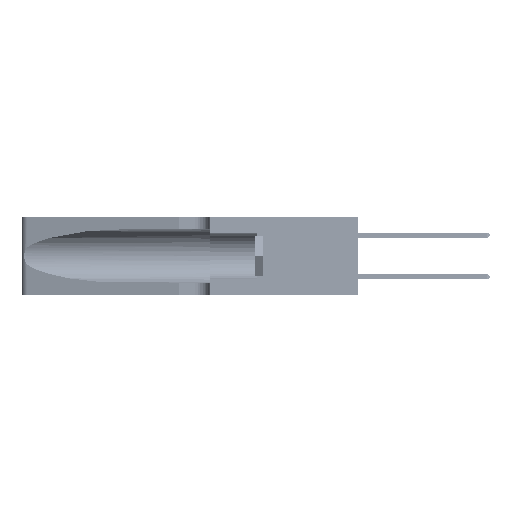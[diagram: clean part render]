
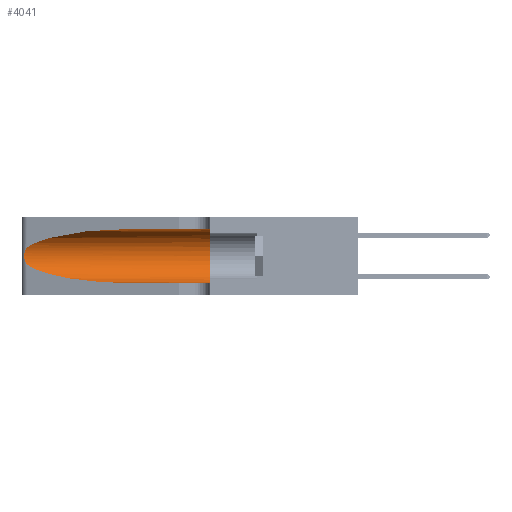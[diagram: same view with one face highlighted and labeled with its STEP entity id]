
A CAD part, left-side view. The second image highlights one B-rep face of the part: STEP entity #4041.
In plain terms, the highlighted cylindrical face has radius 3.308 mm (diameter 6.617 mm), a partial arc.
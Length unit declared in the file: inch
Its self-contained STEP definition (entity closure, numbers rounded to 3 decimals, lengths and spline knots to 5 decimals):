
#20 = DIRECTION ( 'NONE',  ( 0., 0., -1. ) ) ;
#2064 = ORIENTED_EDGE ( 'NONE', *, *, #6880, .T. ) ;
#4041 = ADVANCED_FACE ( 'NONE', ( #22901 ), #19143, .F. ) ;
#5837 = CARTESIAN_POINT ( 'NONE',  ( 0.1305, 0.72297, 0.31525 ) ) ;
#5929 = EDGE_CURVE ( 'NONE', #52014, #38488, #22940, .T. ) ;
#6606 = CARTESIAN_POINT ( 'NONE',  ( 0.25487, 1.22718, 0.14631 ) ) ;
#6880 = EDGE_CURVE ( 'NONE', #41688, #52014, #28350, .T. ) ;
#7652 = DIRECTION ( 'NONE',  ( 0., -1., 0. ) ) ;
#8612 = CARTESIAN_POINT ( 'NONE',  ( 0.25487, 1.22718, 0.22369 ) ) ;
#9420 = DIRECTION ( 'NONE',  ( 0., -1., 0. ) ) ;
#9799 = CARTESIAN_POINT ( 'NONE',  ( 0.25789, 1.23486, 0.15765 ) ) ;
#10320 = CARTESIAN_POINT ( 'NONE',  ( 0.26075, 1.23896, 0.19203 ) ) ;
#10815 = CARTESIAN_POINT ( 'NONE',  ( 0.18966, 0.96281, 0.05475 ) ) ;
#12209 = CARTESIAN_POINT ( 'NONE',  ( 0.1305, 1.61858, 0.185 ) ) ;
#12825 = VECTOR ( 'NONE', #7652, 39.37008 ) ;
#13839 = CARTESIAN_POINT ( 'NONE',  ( 0.25856, 1.23593, 0.16098 ) ) ;
#14347 = CARTESIAN_POINT ( 'NONE',  ( 0.26018, 1.23835, 0.19895 ) ) ;
#14928 = CARTESIAN_POINT ( 'NONE',  ( 0.1305, 0.72297, 0.31525 ) ) ;
#16001 = B_SPLINE_CURVE_WITH_KNOTS ( 'NONE', 3,
 ( #17926, #50094, #34429, #33918, #45875, #14347, #10320, #30403, #26001, #13839, #9799, #37785, #29881, #18095 ),
 .UNSPECIFIED., .F., .F.,
 ( 4, 2, 2, 2, 2, 2, 4 ),
 ( 0., 0.00027, 0.00053, 0.00107, 0.0016, 0.00187, 0.00214 ),
 .UNSPECIFIED. ) ;
#16849 = CARTESIAN_POINT ( 'NONE',  ( 0.1305, 0.35, 0.185 ) ) ;
#17901 = CIRCLE ( 'NONE', #18752, 0.13025 ) ;
#17926 = CARTESIAN_POINT ( 'NONE',  ( 0.25487, 1.22718, 0.22369 ) ) ;
#18095 = CARTESIAN_POINT ( 'NONE',  ( 0.25487, 1.22718, 0.14631 ) ) ;
#18752 = AXIS2_PLACEMENT_3D ( 'NONE', #16849, #25113, #20899 ) ;
#18938 = CARTESIAN_POINT ( 'NONE',  ( 0.25487, 1.22718, 0.14631 ) ) ;
#19143 = CYLINDRICAL_SURFACE ( 'NONE', #37262, 0.13025 ) ;
#20311 = ORIENTED_EDGE ( 'NONE', *, *, #45203, .F. ) ;
#20324 = CARTESIAN_POINT ( 'NONE',  ( 0.1305, 0.72297, 0.05475 ) ) ;
#20899 = DIRECTION ( 'NONE',  ( 0., 0., 1. ) ) ;
#22446 = CARTESIAN_POINT ( 'NONE',  ( 0.1305, 0.35, 0.31525 ) ) ;
#22529 = EDGE_CURVE ( 'NONE', #47591, #37801, #43389, .T. ) ;
#22603 = CARTESIAN_POINT ( 'NONE',  ( 0.2373, 1.15595, 0.08982 ) ) ;
#22784 = CARTESIAN_POINT ( 'NONE',  ( 0.1305, 0.72297, 0.05475 ) ) ;
#22901 = FACE_OUTER_BOUND ( 'NONE', #28384, .T. ) ;
#22940 = LINE ( 'NONE', #32127, #12825 ) ;
#25113 = DIRECTION ( 'NONE',  ( 0., 1., 0. ) ) ;
#25775 = VERTEX_POINT ( 'NONE', #22446 ) ;
#26001 = CARTESIAN_POINT ( 'NONE',  ( 0.26017, 1.23833, 0.17102 ) ) ;
#28350 =( BOUNDED_CURVE ( )  B_SPLINE_CURVE ( 3, ( #18938, #22603, #10815, #22784 ),
 .UNSPECIFIED., .F., .F. ) 
 B_SPLINE_CURVE_WITH_KNOTS ( ( 4, 4 ),
 ( 3.44316, 4.71239 ),
 .UNSPECIFIED. ) 
 CURVE ( )  GEOMETRIC_REPRESENTATION_ITEM ( )  RATIONAL_B_SPLINE_CURVE ( ( 1., 0.87, 0.87, 1. ) ) 
 REPRESENTATION_ITEM ( '' )  );
#28384 = EDGE_LOOP ( 'NONE', ( #28817, #46632, #2064, #51237, #20311, #38474 ) ) ;
#28403 = LINE ( 'NONE', #37052, #37836 ) ;
#28817 = ORIENTED_EDGE ( 'NONE', *, *, #22529, .T. ) ;
#29881 = CARTESIAN_POINT ( 'NONE',  ( 0.25555, 1.22993, 0.14849 ) ) ;
#30403 = CARTESIAN_POINT ( 'NONE',  ( 0.26075, 1.23896, 0.178 ) ) ;
#30963 = CARTESIAN_POINT ( 'NONE',  ( 0.25487, 1.22718, 0.22369 ) ) ;
#32127 = CARTESIAN_POINT ( 'NONE',  ( 0.1305, 1.61858, 0.05475 ) ) ;
#33918 = CARTESIAN_POINT ( 'NONE',  ( 0.25787, 1.23484, 0.2124 ) ) ;
#34429 = CARTESIAN_POINT ( 'NONE',  ( 0.25639, 1.23184, 0.21858 ) ) ;
#37052 = CARTESIAN_POINT ( 'NONE',  ( 0.1305, 1.61858, 0.31525 ) ) ;
#37262 = AXIS2_PLACEMENT_3D ( 'NONE', #12209, #40351, #20 ) ;
#37785 = CARTESIAN_POINT ( 'NONE',  ( 0.25639, 1.23186, 0.15144 ) ) ;
#37801 = VERTEX_POINT ( 'NONE', #8612 ) ;
#37836 = VECTOR ( 'NONE', #9420, 39.37008 ) ;
#38474 = ORIENTED_EDGE ( 'NONE', *, *, #47201, .F. ) ;
#38488 = VERTEX_POINT ( 'NONE', #50607 ) ;
#38681 = CARTESIAN_POINT ( 'NONE',  ( 0.2373, 1.15595, 0.28018 ) ) ;
#40351 = DIRECTION ( 'NONE',  ( 0., -1., 0. ) ) ;
#41550 = EDGE_CURVE ( 'NONE', #37801, #41688, #16001, .T. ) ;
#41688 = VERTEX_POINT ( 'NONE', #6606 ) ;
#43389 =( BOUNDED_CURVE ( )  B_SPLINE_CURVE ( 3, ( #14928, #46613, #38681, #30963 ),
 .UNSPECIFIED., .F., .F. ) 
 B_SPLINE_CURVE_WITH_KNOTS ( ( 4, 4 ),
 ( 1.5708, 2.84003 ),
 .UNSPECIFIED. ) 
 CURVE ( )  GEOMETRIC_REPRESENTATION_ITEM ( )  RATIONAL_B_SPLINE_CURVE ( ( 1., 0.87, 0.87, 1. ) ) 
 REPRESENTATION_ITEM ( '' )  );
#45203 = EDGE_CURVE ( 'NONE', #25775, #38488, #17901, .T. ) ;
#45875 = CARTESIAN_POINT ( 'NONE',  ( 0.25854, 1.2359, 0.20912 ) ) ;
#46613 = CARTESIAN_POINT ( 'NONE',  ( 0.18966, 0.96281, 0.31525 ) ) ;
#46632 = ORIENTED_EDGE ( 'NONE', *, *, #41550, .T. ) ;
#47201 = EDGE_CURVE ( 'NONE', #47591, #25775, #28403, .T. ) ;
#47591 = VERTEX_POINT ( 'NONE', #5837 ) ;
#50094 = CARTESIAN_POINT ( 'NONE',  ( 0.25555, 1.22994, 0.2215 ) ) ;
#50607 = CARTESIAN_POINT ( 'NONE',  ( 0.1305, 0.35, 0.05475 ) ) ;
#51237 = ORIENTED_EDGE ( 'NONE', *, *, #5929, .T. ) ;
#52014 = VERTEX_POINT ( 'NONE', #20324 ) ;
